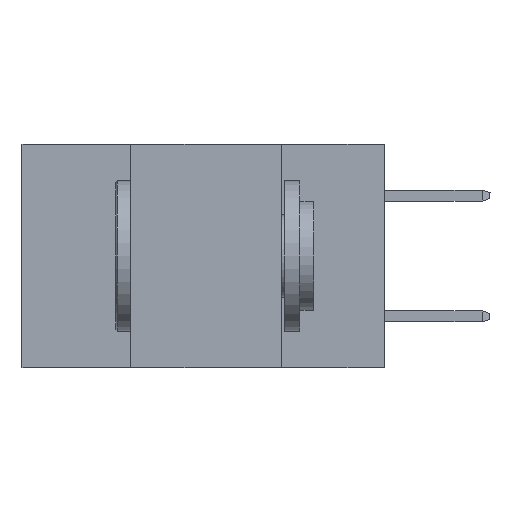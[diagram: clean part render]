
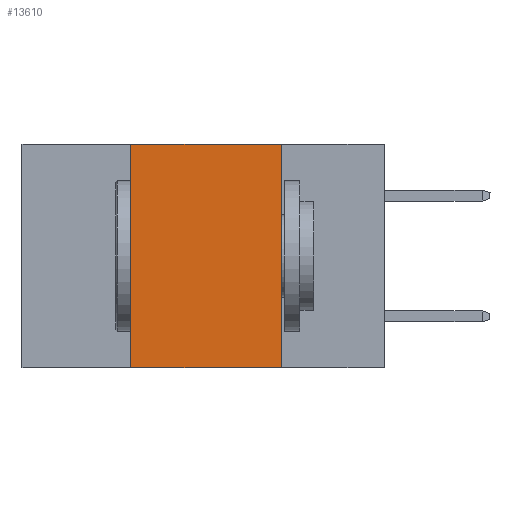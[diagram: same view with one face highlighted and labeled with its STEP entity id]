
A CAD part, left-side view. The second image highlights one B-rep face of the part: STEP entity #13610.
In plain terms, the highlighted planar face has unit normal (-1, 0, 0).
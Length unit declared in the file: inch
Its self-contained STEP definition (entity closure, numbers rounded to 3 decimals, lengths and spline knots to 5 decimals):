
#312 = CARTESIAN_POINT ( 'NONE',  ( 0., 0.42, 0. ) ) ;
#2723 = ORIENTED_EDGE ( 'NONE', *, *, #7233, .F. ) ;
#3419 = DIRECTION ( 'NONE',  ( 1., 0., 0. ) ) ;
#7233 = EDGE_CURVE ( 'NONE', #29431, #7824, #12611, .T. ) ;
#7824 = VERTEX_POINT ( 'NONE', #32519 ) ;
#8484 = VERTEX_POINT ( 'NONE', #16290 ) ;
#8708 = DIRECTION ( 'NONE',  ( 0., 0., -1. ) ) ;
#9043 = DIRECTION ( 'NONE',  ( 0., -1., 0. ) ) ;
#10248 = DIRECTION ( 'NONE',  ( 0., 0., -1. ) ) ;
#10626 = VECTOR ( 'NONE', #10248, 39.37008 ) ;
#12611 = LINE ( 'NONE', #29898, #18660 ) ;
#12859 = CARTESIAN_POINT ( 'NONE',  ( 0., 0.42, 0. ) ) ;
#13610 = ADVANCED_FACE ( 'NONE', ( #30035 ), #29213, .F. ) ;
#13934 = EDGE_CURVE ( 'NONE', #8484, #22728, #27806, .T. ) ;
#14632 = ORIENTED_EDGE ( 'NONE', *, *, #18413, .F. ) ;
#14898 = CARTESIAN_POINT ( 'NONE',  ( 0., 0.6, -0.37 ) ) ;
#15298 = ORIENTED_EDGE ( 'NONE', *, *, #29172, .F. ) ;
#16290 = CARTESIAN_POINT ( 'NONE',  ( 0., 0.42, -0.37 ) ) ;
#16397 = CARTESIAN_POINT ( 'NONE',  ( 0., 0.17, -0.37 ) ) ;
#17905 = CARTESIAN_POINT ( 'NONE',  ( 0., 0.17, 0. ) ) ;
#18363 = DIRECTION ( 'NONE',  ( 0., 0., 1. ) ) ;
#18413 = EDGE_CURVE ( 'NONE', #8484, #29431, #32176, .T. ) ;
#18660 = VECTOR ( 'NONE', #9043, 39.37008 ) ;
#22728 = VERTEX_POINT ( 'NONE', #16397 ) ;
#23678 = VECTOR ( 'NONE', #18363, 39.37008 ) ;
#26997 = VECTOR ( 'NONE', #28400, 39.37008 ) ;
#27806 = LINE ( 'NONE', #14898, #26997 ) ;
#27953 = LINE ( 'NONE', #17905, #10626 ) ;
#28400 = DIRECTION ( 'NONE',  ( 0., -1., 0. ) ) ;
#28693 = ORIENTED_EDGE ( 'NONE', *, *, #13934, .T. ) ;
#29172 = EDGE_CURVE ( 'NONE', #7824, #22728, #27953, .T. ) ;
#29213 = PLANE ( 'NONE',  #30502 ) ;
#29431 = VERTEX_POINT ( 'NONE', #12859 ) ;
#29898 = CARTESIAN_POINT ( 'NONE',  ( 0., 0.6, 0. ) ) ;
#30035 = FACE_OUTER_BOUND ( 'NONE', #33211, .T. ) ;
#30502 = AXIS2_PLACEMENT_3D ( 'NONE', #31715, #3419, #8708 ) ;
#31715 = CARTESIAN_POINT ( 'NONE',  ( 0., 0.6, 0. ) ) ;
#32176 = LINE ( 'NONE', #312, #23678 ) ;
#32519 = CARTESIAN_POINT ( 'NONE',  ( 0., 0.17, 0. ) ) ;
#33211 = EDGE_LOOP ( 'NONE', ( #15298, #2723, #14632, #28693 ) ) ;
